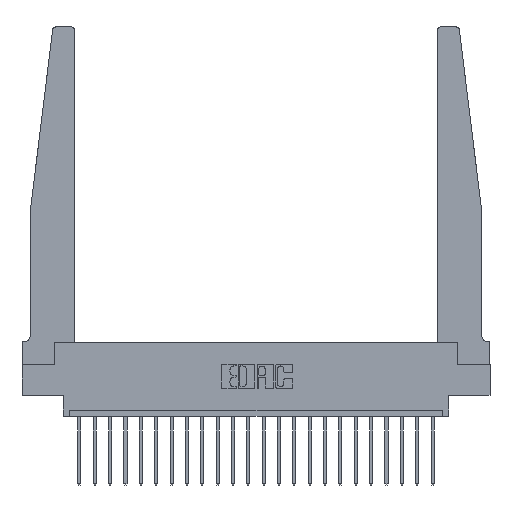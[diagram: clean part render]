
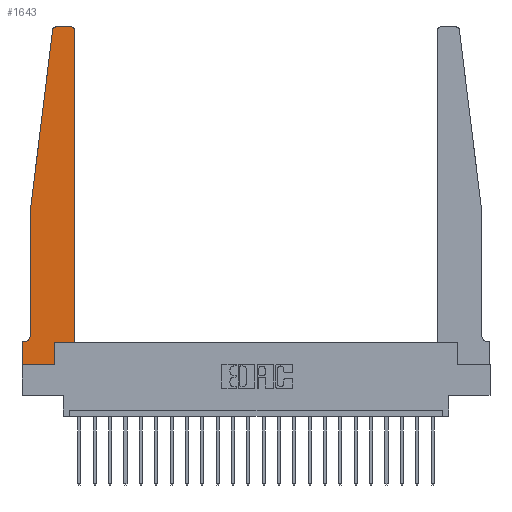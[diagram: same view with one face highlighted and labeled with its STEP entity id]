
A CAD part, top view. The second image highlights one B-rep face of the part: STEP entity #1643.
In plain terms, the highlighted planar face has unit normal (0, 0, 1).
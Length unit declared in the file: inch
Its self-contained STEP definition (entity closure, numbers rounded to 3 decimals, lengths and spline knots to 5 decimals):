
#1 = VERTEX_POINT ( 'NONE', #16258 ) ;
#253 = LINE ( 'NONE', #10224, #9334 ) ;
#748 = ORIENTED_EDGE ( 'NONE', *, *, #15882, .T. ) ;
#1160 = CARTESIAN_POINT ( 'NONE',  ( 0.015, 0.1875, 0.37 ) ) ;
#1398 = CARTESIAN_POINT ( 'NONE',  ( 0.395, 2.72, 0.37 ) ) ;
#1615 = ORIENTED_EDGE ( 'NONE', *, *, #7252, .T. ) ;
#1631 = VECTOR ( 'NONE', #10966, 39.37008 ) ;
#1643 = ADVANCED_FACE ( 'NONE', ( #4972 ), #7607, .T. ) ;
#2116 = CARTESIAN_POINT ( 'NONE',  ( 0.2605, 0.18, 0.37 ) ) ;
#2131 = LINE ( 'NONE', #19116, #20373 ) ;
#2154 = DIRECTION ( 'NONE',  ( 0., 0., 1. ) ) ;
#2243 = EDGE_CURVE ( 'NONE', #13624, #3856, #20769, .T. ) ;
#2312 = DIRECTION ( 'NONE',  ( -1., 0., 0. ) ) ;
#2474 = DIRECTION ( 'NONE',  ( 1., 0., 0. ) ) ;
#2661 = DIRECTION ( 'NONE',  ( 0., -1., 0. ) ) ;
#3106 = EDGE_CURVE ( 'NONE', #18491, #1, #7533, .T. ) ;
#3249 = AXIS2_PLACEMENT_3D ( 'NONE', #7420, #2154, #12638 ) ;
#3730 = ORIENTED_EDGE ( 'NONE', *, *, #8199, .T. ) ;
#3856 = VERTEX_POINT ( 'NONE', #6721 ) ;
#4355 = DIRECTION ( 'NONE',  ( 0., 0., 1. ) ) ;
#4972 = FACE_OUTER_BOUND ( 'NONE', #20609, .T. ) ;
#5532 = EDGE_CURVE ( 'NONE', #20295, #21881, #20083, .T. ) ;
#6173 = VECTOR ( 'NONE', #10872, 39.37008 ) ;
#6292 = ORIENTED_EDGE ( 'NONE', *, *, #5532, .T. ) ;
#6406 = AXIS2_PLACEMENT_3D ( 'NONE', #12570, #21257, #2312 ) ;
#6688 = LINE ( 'NONE', #21432, #1631 ) ;
#6721 = CARTESIAN_POINT ( 'NONE',  ( 0.395, 2.75, 0.37 ) ) ;
#6736 = CARTESIAN_POINT ( 'NONE',  ( 0.425, 2.72, 0.37 ) ) ;
#7037 = CARTESIAN_POINT ( 'NONE',  ( 0., 0.1875, 0.37 ) ) ;
#7252 = EDGE_CURVE ( 'NONE', #18544, #17582, #18923, .T. ) ;
#7420 = CARTESIAN_POINT ( 'NONE',  ( 0.27653, 2.72, 0.37 ) ) ;
#7533 = LINE ( 'NONE', #19756, #13208 ) ;
#7607 = PLANE ( 'NONE',  #16993 ) ;
#7999 = CARTESIAN_POINT ( 'NONE',  ( 0.065, 1.25, 0.37 ) ) ;
#8199 = EDGE_CURVE ( 'NONE', #16356, #18491, #17063, .T. ) ;
#9069 = CARTESIAN_POINT ( 'NONE',  ( 0.065, 0.1875, 0.37 ) ) ;
#9205 = VERTEX_POINT ( 'NONE', #7999 ) ;
#9259 = ORIENTED_EDGE ( 'NONE', *, *, #13807, .T. ) ;
#9334 = VECTOR ( 'NONE', #9592, 39.37008 ) ;
#9592 = DIRECTION ( 'NONE',  ( -1., 0., 0. ) ) ;
#9864 = CARTESIAN_POINT ( 'NONE',  ( 0.24675, 2.72367, 0.37 ) ) ;
#9980 = ORIENTED_EDGE ( 'NONE', *, *, #3106, .T. ) ;
#10224 = CARTESIAN_POINT ( 'NONE',  ( 0.25, 2.75, 0.37 ) ) ;
#10872 = DIRECTION ( 'NONE',  ( 1., 0., 0. ) ) ;
#10966 = DIRECTION ( 'NONE',  ( 0., 1., 0. ) ) ;
#11184 = ORIENTED_EDGE ( 'NONE', *, *, #16167, .T. ) ;
#11373 = CARTESIAN_POINT ( 'NONE',  ( 0.425, 0.18, 0.37 ) ) ;
#12033 = CARTESIAN_POINT ( 'NONE',  ( 0.2605, 0.18, 0.37 ) ) ;
#12213 = DIRECTION ( 'NONE',  ( -0.122, -0.992, 0. ) ) ;
#12249 = CARTESIAN_POINT ( 'NONE',  ( 0.065, 0.2375, 0.37 ) ) ;
#12570 = CARTESIAN_POINT ( 'NONE',  ( 0.015, 0.2375, 0.37 ) ) ;
#12638 = DIRECTION ( 'NONE',  ( 1., 0., 0. ) ) ;
#12969 = CIRCLE ( 'NONE', #6406, 0.05 ) ;
#13166 = DIRECTION ( 'NONE',  ( 1., 0., 0. ) ) ;
#13208 = VECTOR ( 'NONE', #2661, 39.37008 ) ;
#13391 = DIRECTION ( 'NONE',  ( 0., 0., 1. ) ) ;
#13624 = VERTEX_POINT ( 'NONE', #6736 ) ;
#13807 = EDGE_CURVE ( 'NONE', #17582, #13624, #6688, .T. ) ;
#13897 = LINE ( 'NONE', #16173, #20344 ) ;
#14018 = EDGE_CURVE ( 'NONE', #3856, #20295, #253, .T. ) ;
#14332 = CARTESIAN_POINT ( 'NONE',  ( 0.27653, 2.75, 0.37 ) ) ;
#15239 = EDGE_CURVE ( 'NONE', #9205, #19674, #13897, .T. ) ;
#15339 = LINE ( 'NONE', #17958, #6173 ) ;
#15467 = VECTOR ( 'NONE', #2474, 39.37008 ) ;
#15579 = DIRECTION ( 'NONE',  ( 0., 1., 0. ) ) ;
#15882 = EDGE_CURVE ( 'NONE', #17377, #18544, #20948, .T. ) ;
#16167 = EDGE_CURVE ( 'NONE', #1, #17377, #15339, .T. ) ;
#16173 = CARTESIAN_POINT ( 'NONE',  ( 0.065, 1.25, 0.37 ) ) ;
#16258 = CARTESIAN_POINT ( 'NONE',  ( 0., 0., 0.37 ) ) ;
#16356 = VERTEX_POINT ( 'NONE', #1160 ) ;
#16793 = ORIENTED_EDGE ( 'NONE', *, *, #14018, .T. ) ;
#16993 = AXIS2_PLACEMENT_3D ( 'NONE', #19796, #4355, #19647 ) ;
#17063 = LINE ( 'NONE', #9069, #19190 ) ;
#17179 = ORIENTED_EDGE ( 'NONE', *, *, #20918, .T. ) ;
#17377 = VERTEX_POINT ( 'NONE', #18067 ) ;
#17582 = VERTEX_POINT ( 'NONE', #11373 ) ;
#17648 = EDGE_CURVE ( 'NONE', #21881, #9205, #2131, .T. ) ;
#17771 = ORIENTED_EDGE ( 'NONE', *, *, #2243, .T. ) ;
#17958 = CARTESIAN_POINT ( 'NONE',  ( 0., 0., 0.37 ) ) ;
#17967 = ORIENTED_EDGE ( 'NONE', *, *, #15239, .T. ) ;
#18067 = CARTESIAN_POINT ( 'NONE',  ( 0.2605, 0., 0.37 ) ) ;
#18491 = VERTEX_POINT ( 'NONE', #7037 ) ;
#18520 = VECTOR ( 'NONE', #15579, 39.37008 ) ;
#18544 = VERTEX_POINT ( 'NONE', #2116 ) ;
#18923 = LINE ( 'NONE', #21215, #15467 ) ;
#19116 = CARTESIAN_POINT ( 'NONE',  ( 0.065, 1.25, 0.37 ) ) ;
#19190 = VECTOR ( 'NONE', #21166, 39.37008 ) ;
#19647 = DIRECTION ( 'NONE',  ( 1., 0., 0. ) ) ;
#19674 = VERTEX_POINT ( 'NONE', #12249 ) ;
#19756 = CARTESIAN_POINT ( 'NONE',  ( 0., 0., 0.37 ) ) ;
#19796 = CARTESIAN_POINT ( 'NONE',  ( 0., 0.1875, 0.37 ) ) ;
#19967 = DIRECTION ( 'NONE',  ( 0., -1., 0. ) ) ;
#20083 = CIRCLE ( 'NONE', #3249, 0.03 ) ;
#20164 = AXIS2_PLACEMENT_3D ( 'NONE', #1398, #13391, #13166 ) ;
#20295 = VERTEX_POINT ( 'NONE', #14332 ) ;
#20344 = VECTOR ( 'NONE', #19967, 39.37008 ) ;
#20373 = VECTOR ( 'NONE', #12213, 39.37008 ) ;
#20609 = EDGE_LOOP ( 'NONE', ( #16793, #6292, #21016, #17967, #17179, #3730, #9980, #11184, #748, #1615, #9259, #17771 ) ) ;
#20769 = CIRCLE ( 'NONE', #20164, 0.03 ) ;
#20918 = EDGE_CURVE ( 'NONE', #19674, #16356, #12969, .T. ) ;
#20948 = LINE ( 'NONE', #12033, #18520 ) ;
#21016 = ORIENTED_EDGE ( 'NONE', *, *, #17648, .T. ) ;
#21166 = DIRECTION ( 'NONE',  ( -1., 0., 0. ) ) ;
#21215 = CARTESIAN_POINT ( 'NONE',  ( 0.425, 0.18, 0.37 ) ) ;
#21257 = DIRECTION ( 'NONE',  ( 0., 0., -1. ) ) ;
#21432 = CARTESIAN_POINT ( 'NONE',  ( 0.425, 0.18, 0.37 ) ) ;
#21881 = VERTEX_POINT ( 'NONE', #9864 ) ;
